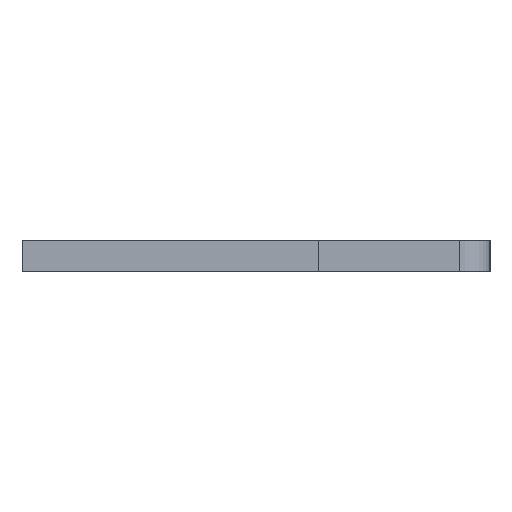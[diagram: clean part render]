
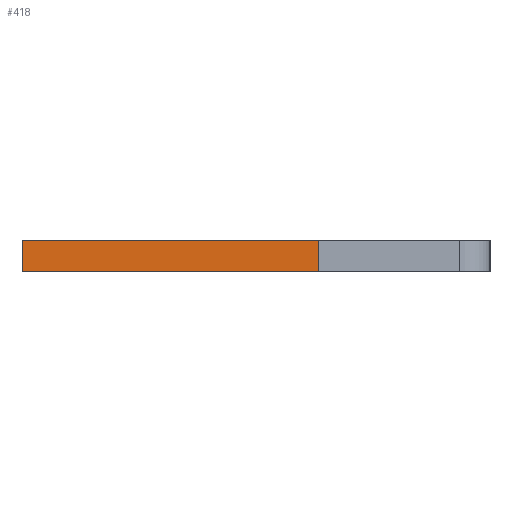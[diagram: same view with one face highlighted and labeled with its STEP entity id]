
A CAD part, left-side view. The second image highlights one B-rep face of the part: STEP entity #418.
In plain terms, the highlighted face is planar.
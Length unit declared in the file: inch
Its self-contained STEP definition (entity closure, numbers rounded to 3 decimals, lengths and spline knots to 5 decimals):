
#94 = FACE_OUTER_BOUND ( 'NONE', #1425, .T. ) ;
#117 = CARTESIAN_POINT ( 'NONE',  ( 0.01, 0.15, -0.04 ) ) ;
#155 = EDGE_CURVE ( 'NONE', #1478, #821, #430, .T. ) ;
#355 = ORIENTED_EDGE ( 'NONE', *, *, #1431, .T. ) ;
#367 = DIRECTION ( 'NONE',  ( 0., 1., 0. ) ) ;
#372 = ORIENTED_EDGE ( 'NONE', *, *, #155, .F. ) ;
#418 = ADVANCED_FACE ( 'NONE', ( #94 ), #766, .F. ) ;
#430 = LINE ( 'NONE', #117, #674 ) ;
#507 = DIRECTION ( 'NONE',  ( 0., 0., 1. ) ) ;
#578 = LINE ( 'NONE', #1168, #1372 ) ;
#609 = LINE ( 'NONE', #782, #910 ) ;
#618 = DIRECTION ( 'NONE',  ( 0., 1., 0. ) ) ;
#656 = EDGE_CURVE ( 'NONE', #821, #1293, #609, .T. ) ;
#663 = DIRECTION ( 'NONE',  ( -1., 0., 0. ) ) ;
#674 = VECTOR ( 'NONE', #367, 39.37008 ) ;
#717 = EDGE_CURVE ( 'NONE', #1478, #973, #578, .T. ) ;
#747 = CARTESIAN_POINT ( 'NONE',  ( 0.01, -0.04, -0.04 ) ) ;
#766 = PLANE ( 'NONE',  #807 ) ;
#782 = CARTESIAN_POINT ( 'NONE',  ( 0.01, 0.15, -0.04 ) ) ;
#807 = AXIS2_PLACEMENT_3D ( 'NONE', #1251, #507, #1376 ) ;
#811 = CARTESIAN_POINT ( 'NONE',  ( -0.01, 0.15, -0.04 ) ) ;
#821 = VERTEX_POINT ( 'NONE', #1045 ) ;
#849 = ORIENTED_EDGE ( 'NONE', *, *, #656, .F. ) ;
#910 = VECTOR ( 'NONE', #1398, 39.37008 ) ;
#973 = VERTEX_POINT ( 'NONE', #1174 ) ;
#995 = ORIENTED_EDGE ( 'NONE', *, *, #717, .T. ) ;
#997 = CARTESIAN_POINT ( 'NONE',  ( -0.01, 0.15, -0.04 ) ) ;
#1045 = CARTESIAN_POINT ( 'NONE',  ( 0.01, 0.15, -0.04 ) ) ;
#1100 = VECTOR ( 'NONE', #618, 39.37008 ) ;
#1168 = CARTESIAN_POINT ( 'NONE',  ( 0.01, -0.04, -0.04 ) ) ;
#1174 = CARTESIAN_POINT ( 'NONE',  ( -0.01, -0.04, -0.04 ) ) ;
#1251 = CARTESIAN_POINT ( 'NONE',  ( 0.01, 0.15, -0.04 ) ) ;
#1293 = VERTEX_POINT ( 'NONE', #811 ) ;
#1372 = VECTOR ( 'NONE', #663, 39.37008 ) ;
#1376 = DIRECTION ( 'NONE',  ( 1., 0., 0. ) ) ;
#1398 = DIRECTION ( 'NONE',  ( -1., 0., 0. ) ) ;
#1425 = EDGE_LOOP ( 'NONE', ( #355, #849, #372, #995 ) ) ;
#1431 = EDGE_CURVE ( 'NONE', #973, #1293, #1433, .T. ) ;
#1433 = LINE ( 'NONE', #997, #1100 ) ;
#1478 = VERTEX_POINT ( 'NONE', #747 ) ;
